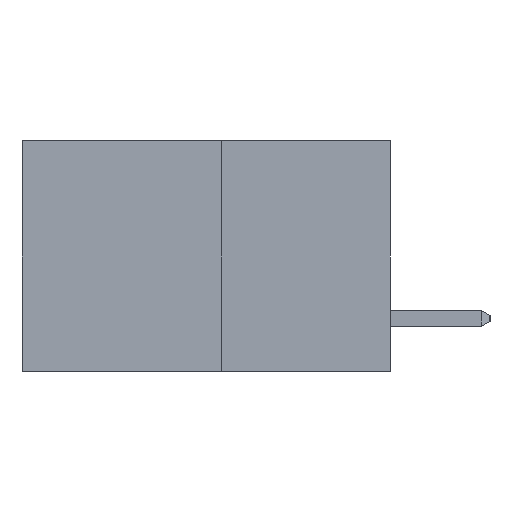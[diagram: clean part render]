
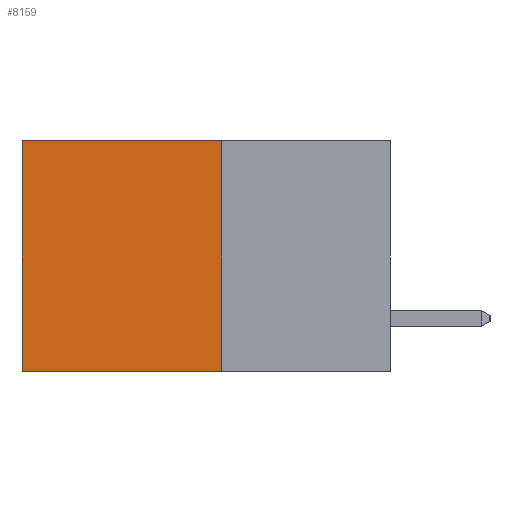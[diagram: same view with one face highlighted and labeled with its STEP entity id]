
A CAD part, left-side view. The second image highlights one B-rep face of the part: STEP entity #8159.
In plain terms, the highlighted planar face has unit normal (-1, 0, 0).
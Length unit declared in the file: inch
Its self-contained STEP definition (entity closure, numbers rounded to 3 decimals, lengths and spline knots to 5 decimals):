
#1072 = CARTESIAN_POINT ( 'NONE',  ( 0.277, 0.27, -0.37 ) ) ;
#1348 = CARTESIAN_POINT ( 'NONE',  ( 0.277, 0.59, -0.37 ) ) ;
#1366 = VERTEX_POINT ( 'NONE', #14582 ) ;
#1413 = VECTOR ( 'NONE', #5218, 39.37008 ) ;
#2397 = ORIENTED_EDGE ( 'NONE', *, *, #3565, .T. ) ;
#2501 = ORIENTED_EDGE ( 'NONE', *, *, #6952, .F. ) ;
#2593 = ORIENTED_EDGE ( 'NONE', *, *, #9457, .F. ) ;
#2596 = CARTESIAN_POINT ( 'NONE',  ( 0.277, 0.27, 0. ) ) ;
#2613 = ORIENTED_EDGE ( 'NONE', *, *, #5181, .T. ) ;
#3147 = DIRECTION ( 'NONE',  ( 0., 1., 0. ) ) ;
#3316 = AXIS2_PLACEMENT_3D ( 'NONE', #15887, #15838, #15812 ) ;
#3565 = EDGE_CURVE ( 'NONE', #8516, #8904, #11764, .T. ) ;
#4490 = VERTEX_POINT ( 'NONE', #10914 ) ;
#5181 = EDGE_CURVE ( 'NONE', #1366, #8516, #9725, .T. ) ;
#5218 = DIRECTION ( 'NONE',  ( 0., 0., -1. ) ) ;
#5385 = EDGE_LOOP ( 'NONE', ( #2397, #2501, #2593, #2613 ) ) ;
#6262 = CARTESIAN_POINT ( 'NONE',  ( 0.277, 0.27, -0.37 ) ) ;
#6906 = VECTOR ( 'NONE', #8922, 39.37008 ) ;
#6952 = EDGE_CURVE ( 'NONE', #4490, #8904, #10455, .T. ) ;
#7093 = VECTOR ( 'NONE', #13071, 39.37008 ) ;
#7162 = CARTESIAN_POINT ( 'NONE',  ( 0.277, 0.59, -0.37 ) ) ;
#7925 = FACE_OUTER_BOUND ( 'NONE', #5385, .T. ) ;
#8079 = LINE ( 'NONE', #1072, #6906 ) ;
#8159 = ADVANCED_FACE ( 'NONE', ( #7925 ), #15927, .F. ) ;
#8516 = VERTEX_POINT ( 'NONE', #12293 ) ;
#8904 = VERTEX_POINT ( 'NONE', #7162 ) ;
#8922 = DIRECTION ( 'NONE',  ( 0., 0., -1. ) ) ;
#9457 = EDGE_CURVE ( 'NONE', #1366, #4490, #8079, .T. ) ;
#9725 = LINE ( 'NONE', #2596, #15836 ) ;
#10455 = LINE ( 'NONE', #6262, #7093 ) ;
#10914 = CARTESIAN_POINT ( 'NONE',  ( 0.277, 0.27, -0.37 ) ) ;
#11764 = LINE ( 'NONE', #1348, #1413 ) ;
#12293 = CARTESIAN_POINT ( 'NONE',  ( 0.277, 0.59, 0. ) ) ;
#13071 = DIRECTION ( 'NONE',  ( 0., 1., 0. ) ) ;
#14582 = CARTESIAN_POINT ( 'NONE',  ( 0.277, 0.27, 0. ) ) ;
#15812 = DIRECTION ( 'NONE',  ( 0., 0., -1. ) ) ;
#15836 = VECTOR ( 'NONE', #3147, 39.37008 ) ;
#15838 = DIRECTION ( 'NONE',  ( 1., 0., 0. ) ) ;
#15887 = CARTESIAN_POINT ( 'NONE',  ( 0.277, 0.27, -0.37 ) ) ;
#15927 = PLANE ( 'NONE',  #3316 ) ;
